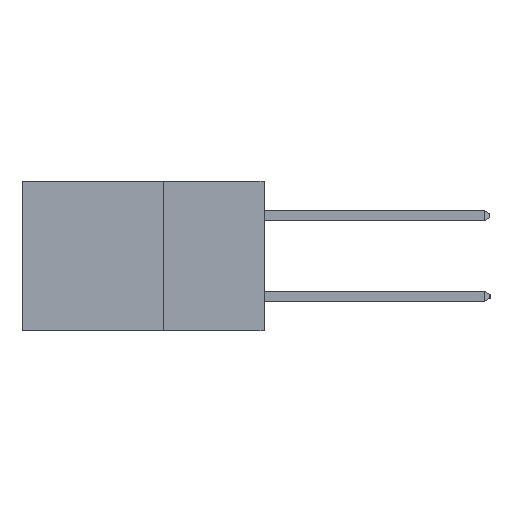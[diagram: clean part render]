
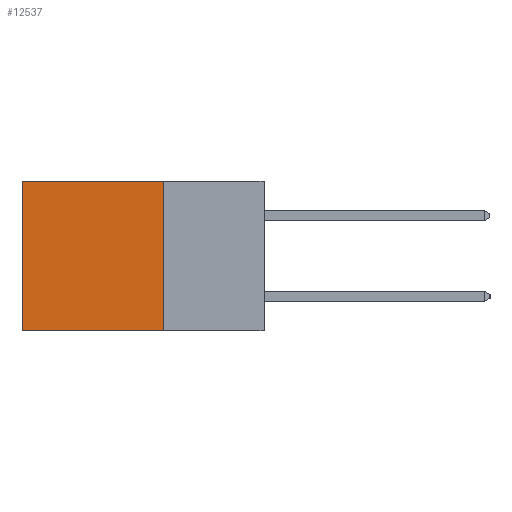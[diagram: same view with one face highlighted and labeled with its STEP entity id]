
A CAD part, left-side view. The second image highlights one B-rep face of the part: STEP entity #12537.
In plain terms, the highlighted planar face has unit normal (-1, 0, 0).
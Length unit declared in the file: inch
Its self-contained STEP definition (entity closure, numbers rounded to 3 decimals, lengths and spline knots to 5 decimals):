
#327 = VERTEX_POINT ( 'NONE', #11675 ) ;
#939 = VERTEX_POINT ( 'NONE', #6580 ) ;
#959 = LINE ( 'NONE', #16586, #11031 ) ;
#1473 = CARTESIAN_POINT ( 'NONE',  ( 0.2615, 0.25, -0.37 ) ) ;
#1529 = AXIS2_PLACEMENT_3D ( 'NONE', #1473, #11457, #2941 ) ;
#1999 = ORIENTED_EDGE ( 'NONE', *, *, #13837, .T. ) ;
#2941 = DIRECTION ( 'NONE',  ( 0., 0., -1. ) ) ;
#3310 = VECTOR ( 'NONE', #8441, 39.37008 ) ;
#3512 = FACE_OUTER_BOUND ( 'NONE', #5350, .T. ) ;
#3661 = EDGE_CURVE ( 'NONE', #15962, #327, #14602, .T. ) ;
#3938 = EDGE_CURVE ( 'NONE', #327, #9203, #13754, .T. ) ;
#3952 = DIRECTION ( 'NONE',  ( 0., 0., -1. ) ) ;
#4284 = DIRECTION ( 'NONE',  ( 0., 1., 0. ) ) ;
#4378 = VECTOR ( 'NONE', #4284, 39.37008 ) ;
#5350 = EDGE_LOOP ( 'NONE', ( #8009, #6800, #9627, #1999 ) ) ;
#6580 = CARTESIAN_POINT ( 'NONE',  ( 0.2615, 0.6, 0. ) ) ;
#6800 = ORIENTED_EDGE ( 'NONE', *, *, #3938, .F. ) ;
#7990 = CARTESIAN_POINT ( 'NONE',  ( 0.2615, 0.25, 0. ) ) ;
#8009 = ORIENTED_EDGE ( 'NONE', *, *, #17765, .T. ) ;
#8441 = DIRECTION ( 'NONE',  ( 0., 0., -1. ) ) ;
#8630 = CARTESIAN_POINT ( 'NONE',  ( 0.2615, 0.25, -0.37 ) ) ;
#9203 = VERTEX_POINT ( 'NONE', #16890 ) ;
#9627 = ORIENTED_EDGE ( 'NONE', *, *, #3661, .F. ) ;
#11031 = VECTOR ( 'NONE', #3952, 39.37008 ) ;
#11457 = DIRECTION ( 'NONE',  ( 1., 0., 0. ) ) ;
#11675 = CARTESIAN_POINT ( 'NONE',  ( 0.2615, 0.25, -0.37 ) ) ;
#12537 = ADVANCED_FACE ( 'NONE', ( #3512 ), #17871, .F. ) ;
#13754 = LINE ( 'NONE', #16624, #16949 ) ;
#13837 = EDGE_CURVE ( 'NONE', #15962, #939, #15601, .T. ) ;
#14159 = CARTESIAN_POINT ( 'NONE',  ( 0.2615, 0.25, 0. ) ) ;
#14602 = LINE ( 'NONE', #8630, #3310 ) ;
#15601 = LINE ( 'NONE', #14159, #4378 ) ;
#15962 = VERTEX_POINT ( 'NONE', #7990 ) ;
#16561 = DIRECTION ( 'NONE',  ( 0., 1., 0. ) ) ;
#16586 = CARTESIAN_POINT ( 'NONE',  ( 0.2615, 0.6, -0.37 ) ) ;
#16624 = CARTESIAN_POINT ( 'NONE',  ( 0.2615, 0.25, -0.37 ) ) ;
#16890 = CARTESIAN_POINT ( 'NONE',  ( 0.2615, 0.6, -0.37 ) ) ;
#16949 = VECTOR ( 'NONE', #16561, 39.37008 ) ;
#17765 = EDGE_CURVE ( 'NONE', #939, #9203, #959, .T. ) ;
#17871 = PLANE ( 'NONE',  #1529 ) ;
